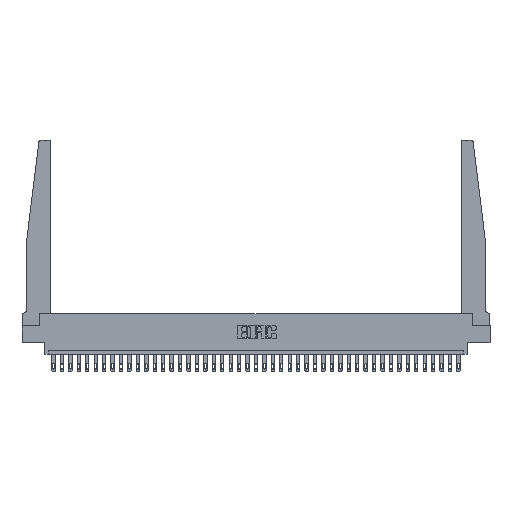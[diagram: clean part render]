
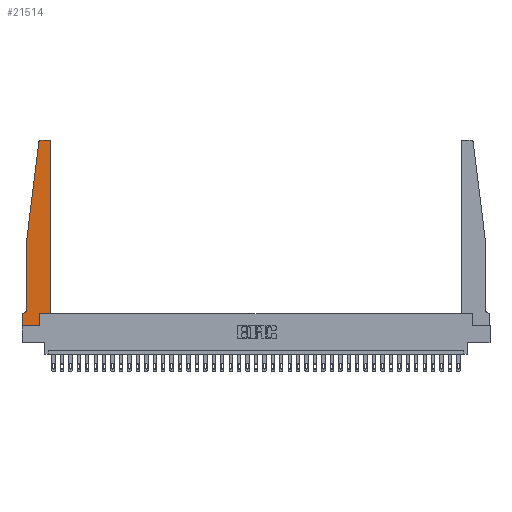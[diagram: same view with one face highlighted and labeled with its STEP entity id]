
A CAD part, top view. The second image highlights one B-rep face of the part: STEP entity #21514.
In plain terms, the highlighted planar face has unit normal (0, 0, 1).
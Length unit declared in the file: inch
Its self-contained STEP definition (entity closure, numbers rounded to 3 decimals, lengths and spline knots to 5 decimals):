
#179 = AXIS2_PLACEMENT_3D ( 'NONE', #18632, #15793, #29344 ) ;
#302 = DIRECTION ( 'NONE',  ( -1., 0., 0. ) ) ;
#543 = VERTEX_POINT ( 'NONE', #20344 ) ;
#1218 = VERTEX_POINT ( 'NONE', #10915 ) ;
#1839 = EDGE_CURVE ( 'NONE', #27138, #2321, #4198, .T. ) ;
#1846 = DIRECTION ( 'NONE',  ( 1., 0., 0. ) ) ;
#2321 = VERTEX_POINT ( 'NONE', #29584 ) ;
#2548 = CARTESIAN_POINT ( 'NONE',  ( 0., 0.1875, 0.37 ) ) ;
#2835 = VERTEX_POINT ( 'NONE', #7367 ) ;
#3296 = EDGE_CURVE ( 'NONE', #26276, #4995, #8723, .T. ) ;
#3715 = CARTESIAN_POINT ( 'NONE',  ( 0.395, 2.72, 0.37 ) ) ;
#4198 = LINE ( 'NONE', #15429, #8694 ) ;
#4598 = CARTESIAN_POINT ( 'NONE',  ( 0.065, 1.25, 0.37 ) ) ;
#4776 = LINE ( 'NONE', #4598, #20662 ) ;
#4995 = VERTEX_POINT ( 'NONE', #6745 ) ;
#5042 = DIRECTION ( 'NONE',  ( 0., 1., 0. ) ) ;
#5047 = ORIENTED_EDGE ( 'NONE', *, *, #33291, .T. ) ;
#5056 = ORIENTED_EDGE ( 'NONE', *, *, #6701, .T. ) ;
#5207 = DIRECTION ( 'NONE',  ( 0., 0., -1. ) ) ;
#5521 = CIRCLE ( 'NONE', #22922, 0.03 ) ;
#5672 = VECTOR ( 'NONE', #30317, 39.37008 ) ;
#5764 = CIRCLE ( 'NONE', #20932, 0.05 ) ;
#6701 = EDGE_CURVE ( 'NONE', #31966, #543, #26204, .T. ) ;
#6745 = CARTESIAN_POINT ( 'NONE',  ( 0., 0.1875, 0.37 ) ) ;
#7067 = ORIENTED_EDGE ( 'NONE', *, *, #15118, .T. ) ;
#7212 = VECTOR ( 'NONE', #12469, 39.37008 ) ;
#7367 = CARTESIAN_POINT ( 'NONE',  ( 0.425, 2.72, 0.37 ) ) ;
#7399 = ORIENTED_EDGE ( 'NONE', *, *, #1839, .T. ) ;
#8566 = VECTOR ( 'NONE', #24289, 39.37008 ) ;
#8694 = VECTOR ( 'NONE', #20572, 39.37008 ) ;
#8723 = LINE ( 'NONE', #24541, #5672 ) ;
#8816 = DIRECTION ( 'NONE',  ( 0., 0., 1. ) ) ;
#10443 = PLANE ( 'NONE',  #25014 ) ;
#10454 = VERTEX_POINT ( 'NONE', #13460 ) ;
#10610 = DIRECTION ( 'NONE',  ( 0., 0., 1. ) ) ;
#10827 = CIRCLE ( 'NONE', #179, 0.03 ) ;
#10915 = CARTESIAN_POINT ( 'NONE',  ( 0.425, 0.18, 0.37 ) ) ;
#11312 = CARTESIAN_POINT ( 'NONE',  ( 0.2605, 0., 0.37 ) ) ;
#11773 = DIRECTION ( 'NONE',  ( 1., 0., 0. ) ) ;
#11783 = VECTOR ( 'NONE', #28214, 39.37008 ) ;
#12233 = VECTOR ( 'NONE', #28832, 39.37008 ) ;
#12469 = DIRECTION ( 'NONE',  ( 1., 0., 0. ) ) ;
#12665 = CARTESIAN_POINT ( 'NONE',  ( 0.065, 1.25, 0.37 ) ) ;
#13460 = CARTESIAN_POINT ( 'NONE',  ( 0.27653, 2.75, 0.37 ) ) ;
#13766 = ORIENTED_EDGE ( 'NONE', *, *, #16714, .T. ) ;
#14047 = EDGE_CURVE ( 'NONE', #31431, #10454, #26386, .T. ) ;
#15031 = LINE ( 'NONE', #33848, #11783 ) ;
#15118 = EDGE_CURVE ( 'NONE', #2835, #31431, #5521, .T. ) ;
#15206 = FACE_OUTER_BOUND ( 'NONE', #31610, .T. ) ;
#15227 = EDGE_CURVE ( 'NONE', #30567, #27138, #23396, .T. ) ;
#15429 = CARTESIAN_POINT ( 'NONE',  ( 0.2605, 0.18, 0.37 ) ) ;
#15793 = DIRECTION ( 'NONE',  ( 0., 0., 1. ) ) ;
#15825 = CARTESIAN_POINT ( 'NONE',  ( 0.25, 2.75, 0.37 ) ) ;
#15906 = EDGE_CURVE ( 'NONE', #1218, #2835, #21594, .T. ) ;
#16327 = ORIENTED_EDGE ( 'NONE', *, *, #3296, .T. ) ;
#16714 = EDGE_CURVE ( 'NONE', #10454, #31966, #10827, .T. ) ;
#17425 = CARTESIAN_POINT ( 'NONE',  ( 0.065, 0.2375, 0.37 ) ) ;
#17435 = EDGE_CURVE ( 'NONE', #2321, #1218, #15031, .T. ) ;
#18150 = DIRECTION ( 'NONE',  ( 0., -1., 0. ) ) ;
#18246 = CARTESIAN_POINT ( 'NONE',  ( 0.425, 0.18, 0.37 ) ) ;
#18632 = CARTESIAN_POINT ( 'NONE',  ( 0.27653, 2.72, 0.37 ) ) ;
#18922 = ORIENTED_EDGE ( 'NONE', *, *, #14047, .T. ) ;
#19490 = LINE ( 'NONE', #19661, #21737 ) ;
#19661 = CARTESIAN_POINT ( 'NONE',  ( 0., 0., 0.37 ) ) ;
#20344 = CARTESIAN_POINT ( 'NONE',  ( 0.065, 1.25, 0.37 ) ) ;
#20572 = DIRECTION ( 'NONE',  ( 0., 1., 0. ) ) ;
#20662 = VECTOR ( 'NONE', #18150, 39.37008 ) ;
#20932 = AXIS2_PLACEMENT_3D ( 'NONE', #34727, #5207, #302 ) ;
#21514 = ADVANCED_FACE ( 'NONE', ( #15206 ), #10443, .T. ) ;
#21594 = LINE ( 'NONE', #18246, #34211 ) ;
#21737 = VECTOR ( 'NONE', #24412, 39.37008 ) ;
#22922 = AXIS2_PLACEMENT_3D ( 'NONE', #3715, #8816, #11773 ) ;
#23163 = EDGE_CURVE ( 'NONE', #4995, #30567, #19490, .T. ) ;
#23396 = LINE ( 'NONE', #34101, #7212 ) ;
#23742 = EDGE_CURVE ( 'NONE', #543, #33668, #4776, .T. ) ;
#23777 = ORIENTED_EDGE ( 'NONE', *, *, #17435, .T. ) ;
#24289 = DIRECTION ( 'NONE',  ( -1., 0., 0. ) ) ;
#24412 = DIRECTION ( 'NONE',  ( 0., -1., 0. ) ) ;
#24541 = CARTESIAN_POINT ( 'NONE',  ( 0.065, 0.1875, 0.37 ) ) ;
#25014 = AXIS2_PLACEMENT_3D ( 'NONE', #2548, #10610, #1846 ) ;
#26204 = LINE ( 'NONE', #12665, #12233 ) ;
#26276 = VERTEX_POINT ( 'NONE', #33147 ) ;
#26386 = LINE ( 'NONE', #15825, #8566 ) ;
#27078 = ORIENTED_EDGE ( 'NONE', *, *, #23163, .T. ) ;
#27138 = VERTEX_POINT ( 'NONE', #11312 ) ;
#28214 = DIRECTION ( 'NONE',  ( 1., 0., 0. ) ) ;
#28832 = DIRECTION ( 'NONE',  ( -0.122, -0.992, 0. ) ) ;
#28910 = ORIENTED_EDGE ( 'NONE', *, *, #15906, .T. ) ;
#29344 = DIRECTION ( 'NONE',  ( 1., 0., 0. ) ) ;
#29584 = CARTESIAN_POINT ( 'NONE',  ( 0.2605, 0.18, 0.37 ) ) ;
#29726 = CARTESIAN_POINT ( 'NONE',  ( 0., 0., 0.37 ) ) ;
#30317 = DIRECTION ( 'NONE',  ( -1., 0., 0. ) ) ;
#30408 = CARTESIAN_POINT ( 'NONE',  ( 0.395, 2.75, 0.37 ) ) ;
#30505 = ORIENTED_EDGE ( 'NONE', *, *, #15227, .T. ) ;
#30567 = VERTEX_POINT ( 'NONE', #29726 ) ;
#31431 = VERTEX_POINT ( 'NONE', #30408 ) ;
#31526 = ORIENTED_EDGE ( 'NONE', *, *, #23742, .T. ) ;
#31610 = EDGE_LOOP ( 'NONE', ( #18922, #13766, #5056, #31526, #5047, #16327, #27078, #30505, #7399, #23777, #28910, #7067 ) ) ;
#31966 = VERTEX_POINT ( 'NONE', #34008 ) ;
#33147 = CARTESIAN_POINT ( 'NONE',  ( 0.015, 0.1875, 0.37 ) ) ;
#33291 = EDGE_CURVE ( 'NONE', #33668, #26276, #5764, .T. ) ;
#33668 = VERTEX_POINT ( 'NONE', #17425 ) ;
#33848 = CARTESIAN_POINT ( 'NONE',  ( 0.425, 0.18, 0.37 ) ) ;
#34008 = CARTESIAN_POINT ( 'NONE',  ( 0.24675, 2.72367, 0.37 ) ) ;
#34101 = CARTESIAN_POINT ( 'NONE',  ( 0., 0., 0.37 ) ) ;
#34211 = VECTOR ( 'NONE', #5042, 39.37008 ) ;
#34727 = CARTESIAN_POINT ( 'NONE',  ( 0.015, 0.2375, 0.37 ) ) ;
